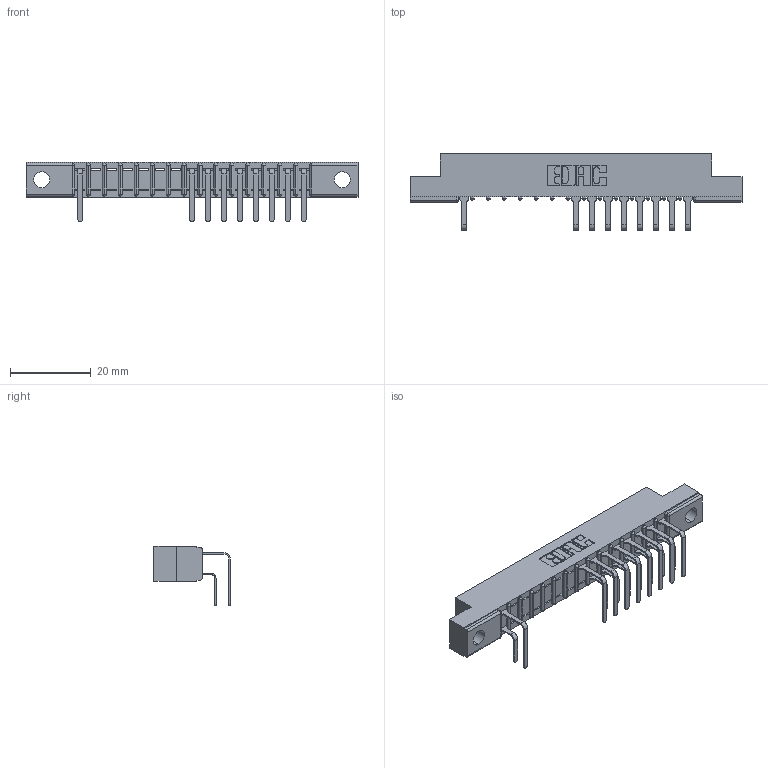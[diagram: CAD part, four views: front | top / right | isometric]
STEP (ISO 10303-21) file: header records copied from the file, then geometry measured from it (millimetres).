
FILE_DESCRIPTION (( 'STEP AP203' ), '1' );
FILE_NAME ('307-030-558-204.STEP', '2018-08-04T19:52:16', ( '' ), ( '' ), 'SwSTEP 2.0', 'SolidWorks 2016', '' );
FILE_SCHEMA (( 'CONFIG_CONTROL_DESIGN' ));
Length unit declared in the file: inch
Products named in the file (4): 307 Part_.156 Dia Mounting Holes; 307-290-001_558 559 - 1 (Single); 307-290-001_558 - 2 (Single); 307-030-558-204
Assembly tree (18 placements, depth 2):
  307-030-558-204
    307 Part_.156 Dia Mounting Holes
    307-290-001_558 559 - 1 (Single)  x8
    307-290-001_558 - 2 (Single)  x9
Bounding box: 82.45 x 18.96 x 14.81 mm (x, y, z)
Volume: 5196.5 mm3; surface area: 8142 mm2
Topology: 18 solids, 18 shells, 1128 faces, 3189 edges, 2058 vertices
Faces by surface type: plane 723, cylinder 373, sphere 32
Entity records: 18117 total; most frequent: CARTESIAN_POINT 3034, ORIENTED_EDGE 3014, DIRECTION 2961, EDGE_CURVE 1507, VECTOR 1151, LINE 1151, VERTEX_POINT 978, AXIS2_PLACEMENT_3D 905
